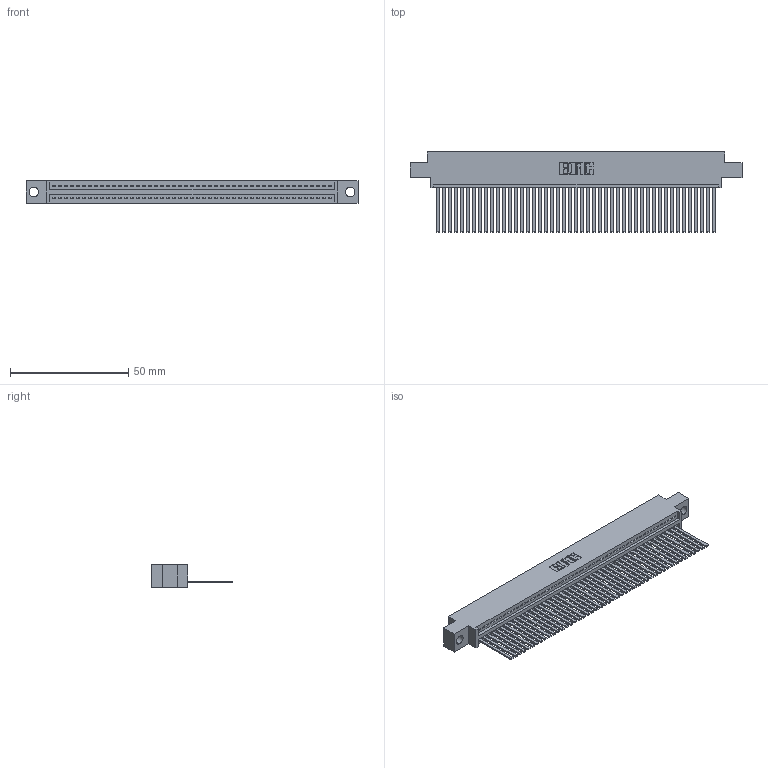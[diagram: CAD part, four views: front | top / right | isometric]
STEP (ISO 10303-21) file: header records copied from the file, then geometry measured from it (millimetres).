
FILE_DESCRIPTION (( 'STEP AP203' ), '1' );
FILE_NAME ('345-047-544-604.STEP', '2018-09-10T15:50:36', ( '' ), ( '' ), 'SwSTEP 2.0', 'SolidWorks 2016', '' );
FILE_SCHEMA (( 'CONFIG_CONTROL_DESIGN' ));
Length unit declared in the file: inch
Products named in the file (3): 345-047-544-604; 345 Part_0.170 Offset - 0.156 Dia-TH; 345-292-001_345-293-144
Assembly tree (48 placements, depth 2):
  345-047-544-604
    345 Part_0.170 Offset - 0.156 Dia-TH
    345-292-001_345-293-144  x47
Bounding box: 140.59 x 33.96 x 9.4 mm (x, y, z)
Volume: 13737.3 mm3; surface area: 19893 mm2
Topology: 48 solids, 48 shells, 2574 faces, 7779 edges, 5122 vertices
Faces by surface type: plane 1776, cylinder 798
Entity records: 34651 total; most frequent: CARTESIAN_POINT 6009, ORIENTED_EDGE 5990, DIRECTION 5237, EDGE_CURVE 2995, LINE 2679, VECTOR 2679, VERTEX_POINT 1994, AXIS2_PLACEMENT_3D 1279
